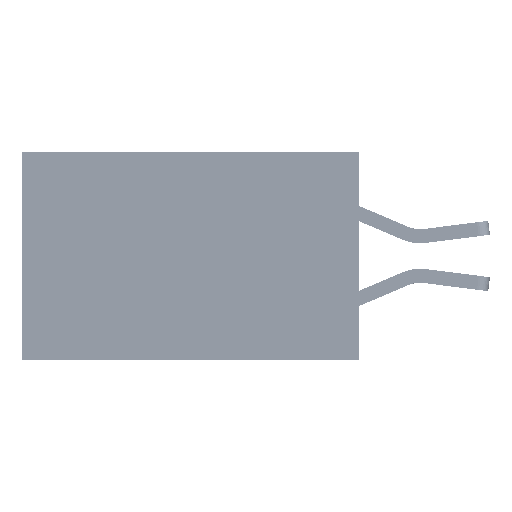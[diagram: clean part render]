
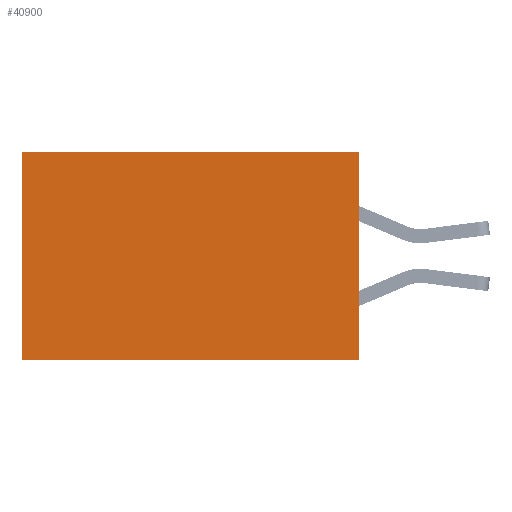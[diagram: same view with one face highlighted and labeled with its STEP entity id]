
A CAD part, left-side view. The second image highlights one B-rep face of the part: STEP entity #40900.
In plain terms, the highlighted planar face has unit normal (-1, 0, 0).
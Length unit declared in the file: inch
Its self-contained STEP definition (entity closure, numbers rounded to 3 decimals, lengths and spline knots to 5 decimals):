
#223 = VECTOR ( 'NONE', #20857, 39.37008 ) ;
#813 = AXIS2_PLACEMENT_3D ( 'NONE', #35067, #7148, #31677 ) ;
#1945 = EDGE_CURVE ( 'NONE', #37597, #44896, #20092, .T. ) ;
#6644 = FACE_OUTER_BOUND ( 'NONE', #9987, .T. ) ;
#6837 = PLANE ( 'NONE',  #813 ) ;
#7148 = DIRECTION ( 'NONE',  ( 1., 0., 0. ) ) ;
#9987 = EDGE_LOOP ( 'NONE', ( #40158, #40938, #15440, #30793 ) ) ;
#10686 = CARTESIAN_POINT ( 'NONE',  ( 0.2875, 0.6, 0. ) ) ;
#11975 = CARTESIAN_POINT ( 'NONE',  ( 0.2875, 0., 0. ) ) ;
#14041 = VERTEX_POINT ( 'NONE', #10686 ) ;
#15245 = DIRECTION ( 'NONE',  ( 0., 0., -1. ) ) ;
#15440 = ORIENTED_EDGE ( 'NONE', *, *, #40515, .F. ) ;
#18367 = VECTOR ( 'NONE', #15245, 39.37008 ) ;
#18893 = VECTOR ( 'NONE', #32072, 39.37008 ) ;
#19398 = EDGE_CURVE ( 'NONE', #14041, #44896, #37235, .T. ) ;
#20092 = LINE ( 'NONE', #25743, #28411 ) ;
#20857 = DIRECTION ( 'NONE',  ( 0., 1., 0. ) ) ;
#23424 = CARTESIAN_POINT ( 'NONE',  ( 0.2875, 0., 0. ) ) ;
#25743 = CARTESIAN_POINT ( 'NONE',  ( 0.2875, 0., -0.37 ) ) ;
#26601 = CARTESIAN_POINT ( 'NONE',  ( 0.2875, 0., -0.37 ) ) ;
#28411 = VECTOR ( 'NONE', #40625, 39.37008 ) ;
#28924 = LINE ( 'NONE', #11975, #18367 ) ;
#29859 = EDGE_CURVE ( 'NONE', #34453, #14041, #41877, .T. ) ;
#30793 = ORIENTED_EDGE ( 'NONE', *, *, #29859, .T. ) ;
#31677 = DIRECTION ( 'NONE',  ( 0., 0., -1. ) ) ;
#32072 = DIRECTION ( 'NONE',  ( 0., 0., -1. ) ) ;
#34453 = VERTEX_POINT ( 'NONE', #23424 ) ;
#34942 = CARTESIAN_POINT ( 'NONE',  ( 0.2875, 0., 0. ) ) ;
#35067 = CARTESIAN_POINT ( 'NONE',  ( 0.2875, 0., 0. ) ) ;
#35459 = CARTESIAN_POINT ( 'NONE',  ( 0.2875, 0.6, 0. ) ) ;
#37235 = LINE ( 'NONE', #35459, #18893 ) ;
#37597 = VERTEX_POINT ( 'NONE', #26601 ) ;
#40158 = ORIENTED_EDGE ( 'NONE', *, *, #19398, .T. ) ;
#40515 = EDGE_CURVE ( 'NONE', #34453, #37597, #28924, .T. ) ;
#40625 = DIRECTION ( 'NONE',  ( 0., 1., 0. ) ) ;
#40900 = ADVANCED_FACE ( 'NONE', ( #6644 ), #6837, .F. ) ;
#40938 = ORIENTED_EDGE ( 'NONE', *, *, #1945, .F. ) ;
#41877 = LINE ( 'NONE', #34942, #223 ) ;
#43717 = CARTESIAN_POINT ( 'NONE',  ( 0.2875, 0.6, -0.37 ) ) ;
#44896 = VERTEX_POINT ( 'NONE', #43717 ) ;
